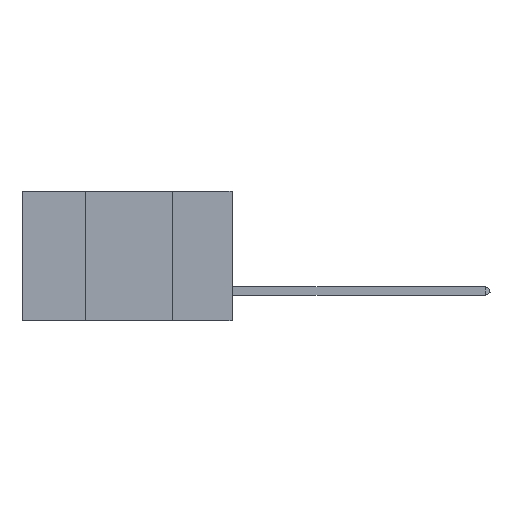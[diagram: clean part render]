
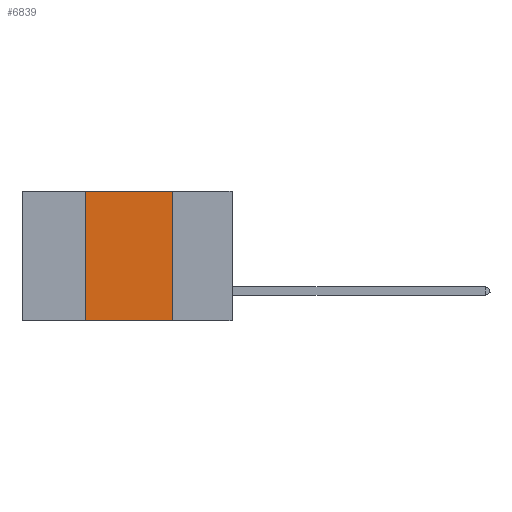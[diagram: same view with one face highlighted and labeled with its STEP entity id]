
A CAD part, left-side view. The second image highlights one B-rep face of the part: STEP entity #6839.
In plain terms, the highlighted planar face has unit normal (-1, 0, 0).
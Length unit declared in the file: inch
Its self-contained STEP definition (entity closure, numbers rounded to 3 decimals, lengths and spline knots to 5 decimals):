
#240 = VERTEX_POINT ( 'NONE', #4716 ) ;
#1332 = CARTESIAN_POINT ( 'NONE',  ( 0., 0.6, 0. ) ) ;
#2373 = ORIENTED_EDGE ( 'NONE', *, *, #6265, .F. ) ;
#2739 = EDGE_CURVE ( 'NONE', #15317, #240, #19467, .T. ) ;
#3193 = ORIENTED_EDGE ( 'NONE', *, *, #19704, .F. ) ;
#4716 = CARTESIAN_POINT ( 'NONE',  ( 0., 0.17, -0.37 ) ) ;
#4774 = DIRECTION ( 'NONE',  ( 0., -1., 0. ) ) ;
#5405 = DIRECTION ( 'NONE',  ( 0., 0., -1. ) ) ;
#5865 = AXIS2_PLACEMENT_3D ( 'NONE', #21098, #11575, #15540 ) ;
#6265 = EDGE_CURVE ( 'NONE', #15701, #15317, #8961, .T. ) ;
#6839 = ADVANCED_FACE ( 'NONE', ( #12739 ), #11657, .F. ) ;
#7561 = LINE ( 'NONE', #9268, #15470 ) ;
#7880 = VERTEX_POINT ( 'NONE', #8444 ) ;
#8444 = CARTESIAN_POINT ( 'NONE',  ( 0., 0.42, -0.37 ) ) ;
#8961 = LINE ( 'NONE', #1332, #20973 ) ;
#9139 = EDGE_LOOP ( 'NONE', ( #13939, #2373, #3193, #23111 ) ) ;
#9268 = CARTESIAN_POINT ( 'NONE',  ( 0., 0.42, 0. ) ) ;
#9814 = VECTOR ( 'NONE', #23595, 39.37008 ) ;
#10098 = LINE ( 'NONE', #21694, #9814 ) ;
#11256 = VECTOR ( 'NONE', #5405, 39.37008 ) ;
#11575 = DIRECTION ( 'NONE',  ( 1., 0., 0. ) ) ;
#11657 = PLANE ( 'NONE',  #5865 ) ;
#12739 = FACE_OUTER_BOUND ( 'NONE', #9139, .T. ) ;
#13066 = CARTESIAN_POINT ( 'NONE',  ( 0., 0.17, 0. ) ) ;
#13939 = ORIENTED_EDGE ( 'NONE', *, *, #2739, .F. ) ;
#15317 = VERTEX_POINT ( 'NONE', #13066 ) ;
#15470 = VECTOR ( 'NONE', #22182, 39.37008 ) ;
#15540 = DIRECTION ( 'NONE',  ( 0., 0., -1. ) ) ;
#15701 = VERTEX_POINT ( 'NONE', #21940 ) ;
#18394 = CARTESIAN_POINT ( 'NONE',  ( 0., 0.17, 0. ) ) ;
#19467 = LINE ( 'NONE', #18394, #11256 ) ;
#19704 = EDGE_CURVE ( 'NONE', #7880, #15701, #7561, .T. ) ;
#20973 = VECTOR ( 'NONE', #4774, 39.37008 ) ;
#21098 = CARTESIAN_POINT ( 'NONE',  ( 0., 0.6, 0. ) ) ;
#21489 = EDGE_CURVE ( 'NONE', #7880, #240, #10098, .T. ) ;
#21694 = CARTESIAN_POINT ( 'NONE',  ( 0., 0.6, -0.37 ) ) ;
#21940 = CARTESIAN_POINT ( 'NONE',  ( 0., 0.42, 0. ) ) ;
#22182 = DIRECTION ( 'NONE',  ( 0., 0., 1. ) ) ;
#23111 = ORIENTED_EDGE ( 'NONE', *, *, #21489, .T. ) ;
#23595 = DIRECTION ( 'NONE',  ( 0., -1., 0. ) ) ;
